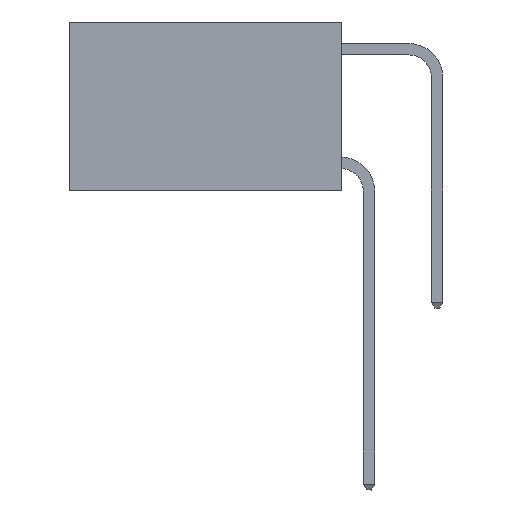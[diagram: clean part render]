
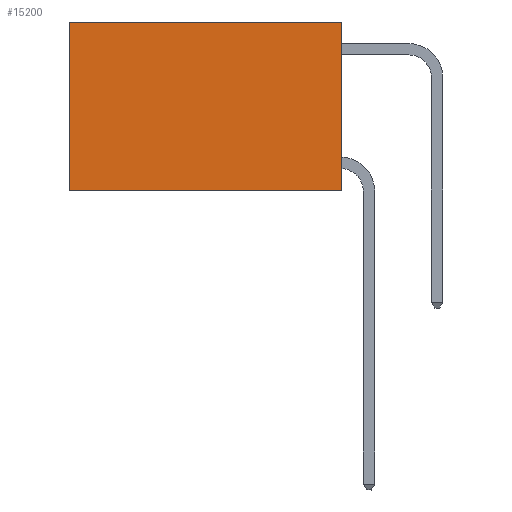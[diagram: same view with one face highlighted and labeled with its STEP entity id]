
A CAD part, left-side view. The second image highlights one B-rep face of the part: STEP entity #15200.
In plain terms, the highlighted planar face has unit normal (-1, 0, 0).
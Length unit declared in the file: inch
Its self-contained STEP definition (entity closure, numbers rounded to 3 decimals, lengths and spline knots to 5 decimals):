
#775 = VERTEX_POINT ( 'NONE', #5403 ) ;
#965 = CARTESIAN_POINT ( 'NONE',  ( 0.2625, 0., 0. ) ) ;
#987 = CARTESIAN_POINT ( 'NONE',  ( 0.2625, 0., -0.37 ) ) ;
#1502 = CARTESIAN_POINT ( 'NONE',  ( 0.2625, 0.6, 0. ) ) ;
#1864 = LINE ( 'NONE', #987, #18138 ) ;
#2720 = EDGE_CURVE ( 'NONE', #5134, #775, #3082, .T. ) ;
#3013 = DIRECTION ( 'NONE',  ( 0., 0., -1. ) ) ;
#3082 = LINE ( 'NONE', #22095, #3727 ) ;
#3343 = EDGE_CURVE ( 'NONE', #4120, #10219, #20271, .T. ) ;
#3727 = VECTOR ( 'NONE', #24129, 39.37008 ) ;
#4120 = VERTEX_POINT ( 'NONE', #17792 ) ;
#4369 = ORIENTED_EDGE ( 'NONE', *, *, #2720, .F. ) ;
#5134 = VERTEX_POINT ( 'NONE', #17146 ) ;
#5403 = CARTESIAN_POINT ( 'NONE',  ( 0.2625, 0., -0.37 ) ) ;
#6004 = EDGE_CURVE ( 'NONE', #5134, #4120, #12476, .T. ) ;
#9804 = CARTESIAN_POINT ( 'NONE',  ( 0.2625, 0., 0. ) ) ;
#10219 = VERTEX_POINT ( 'NONE', #13067 ) ;
#10781 = EDGE_CURVE ( 'NONE', #775, #10219, #1864, .T. ) ;
#11844 = DIRECTION ( 'NONE',  ( 0., 1., 0. ) ) ;
#12024 = ORIENTED_EDGE ( 'NONE', *, *, #6004, .T. ) ;
#12476 = LINE ( 'NONE', #9804, #22664 ) ;
#13067 = CARTESIAN_POINT ( 'NONE',  ( 0.2625, 0.6, -0.37 ) ) ;
#15200 = ADVANCED_FACE ( 'NONE', ( #17950 ), #23322, .F. ) ;
#15262 = DIRECTION ( 'NONE',  ( 1., 0., 0. ) ) ;
#15286 = DIRECTION ( 'NONE',  ( 0., 1., 0. ) ) ;
#15515 = VECTOR ( 'NONE', #21814, 39.37008 ) ;
#16400 = ORIENTED_EDGE ( 'NONE', *, *, #10781, .F. ) ;
#17146 = CARTESIAN_POINT ( 'NONE',  ( 0.2625, 0., 0. ) ) ;
#17792 = CARTESIAN_POINT ( 'NONE',  ( 0.2625, 0.6, 0. ) ) ;
#17950 = FACE_OUTER_BOUND ( 'NONE', #18699, .T. ) ;
#18138 = VECTOR ( 'NONE', #15286, 39.37008 ) ;
#18699 = EDGE_LOOP ( 'NONE', ( #25562, #16400, #4369, #12024 ) ) ;
#18817 = AXIS2_PLACEMENT_3D ( 'NONE', #965, #15262, #3013 ) ;
#20271 = LINE ( 'NONE', #1502, #15515 ) ;
#21814 = DIRECTION ( 'NONE',  ( 0., 0., -1. ) ) ;
#22095 = CARTESIAN_POINT ( 'NONE',  ( 0.2625, 0., 0. ) ) ;
#22664 = VECTOR ( 'NONE', #11844, 39.37008 ) ;
#23322 = PLANE ( 'NONE',  #18817 ) ;
#24129 = DIRECTION ( 'NONE',  ( 0., 0., -1. ) ) ;
#25562 = ORIENTED_EDGE ( 'NONE', *, *, #3343, .T. ) ;
